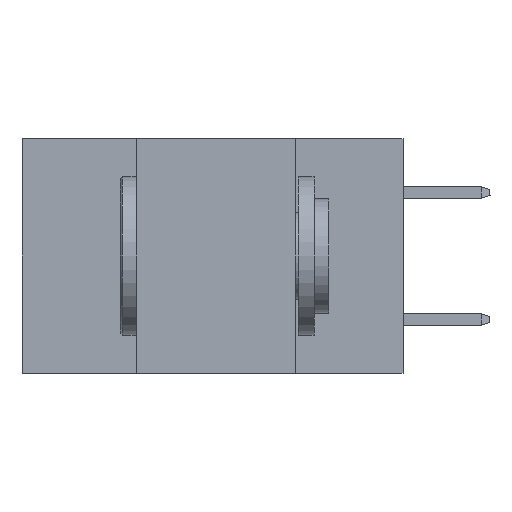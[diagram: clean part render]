
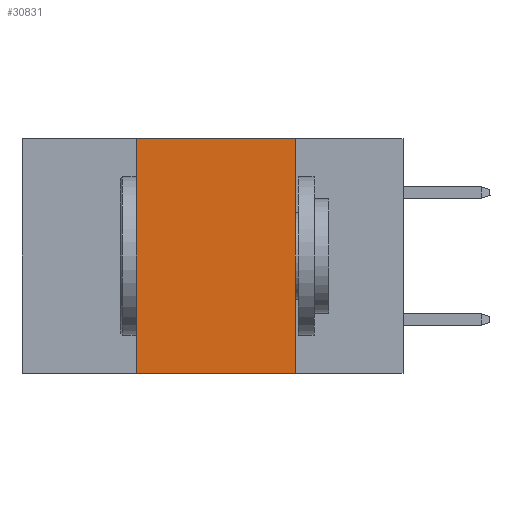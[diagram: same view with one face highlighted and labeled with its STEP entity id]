
A CAD part, left-side view. The second image highlights one B-rep face of the part: STEP entity #30831.
In plain terms, the highlighted planar face has unit normal (-1, 0, 0).
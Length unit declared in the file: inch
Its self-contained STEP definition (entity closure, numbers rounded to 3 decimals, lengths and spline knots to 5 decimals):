
#2144 = DIRECTION ( 'NONE',  ( 0., -1., 0. ) ) ;
#2482 = CARTESIAN_POINT ( 'NONE',  ( 0., 0.6, 0. ) ) ;
#2687 = DIRECTION ( 'NONE',  ( 1., 0., 0. ) ) ;
#2894 = PLANE ( 'NONE',  #32822 ) ;
#4077 = VECTOR ( 'NONE', #2144, 39.37008 ) ;
#4418 = CARTESIAN_POINT ( 'NONE',  ( 0., 0.17, -0.37 ) ) ;
#5688 = DIRECTION ( 'NONE',  ( 0., 0., 1. ) ) ;
#5837 = VECTOR ( 'NONE', #7224, 39.37008 ) ;
#6856 = EDGE_CURVE ( 'NONE', #21962, #34733, #12440, .T. ) ;
#7224 = DIRECTION ( 'NONE',  ( 0., 0., -1. ) ) ;
#7876 = CARTESIAN_POINT ( 'NONE',  ( 0., 0.6, -0.37 ) ) ;
#8128 = EDGE_CURVE ( 'NONE', #21962, #21107, #26295, .T. ) ;
#8427 = FACE_OUTER_BOUND ( 'NONE', #31121, .T. ) ;
#9967 = CARTESIAN_POINT ( 'NONE',  ( 0., 0.17, 0. ) ) ;
#10916 = ORIENTED_EDGE ( 'NONE', *, *, #25768, .F. ) ;
#11993 = ORIENTED_EDGE ( 'NONE', *, *, #35863, .F. ) ;
#12440 = LINE ( 'NONE', #18396, #23446 ) ;
#13232 = CARTESIAN_POINT ( 'NONE',  ( 0., 0.42, -0.37 ) ) ;
#16250 = LINE ( 'NONE', #25644, #5837 ) ;
#18396 = CARTESIAN_POINT ( 'NONE',  ( 0., 0.42, 0. ) ) ;
#18605 = LINE ( 'NONE', #37562, #29808 ) ;
#21107 = VERTEX_POINT ( 'NONE', #4418 ) ;
#21135 = DIRECTION ( 'NONE',  ( 0., 0., -1. ) ) ;
#21881 = DIRECTION ( 'NONE',  ( 0., -1., 0. ) ) ;
#21962 = VERTEX_POINT ( 'NONE', #13232 ) ;
#22033 = VERTEX_POINT ( 'NONE', #9967 ) ;
#23446 = VECTOR ( 'NONE', #5688, 39.37008 ) ;
#25644 = CARTESIAN_POINT ( 'NONE',  ( 0., 0.17, 0. ) ) ;
#25768 = EDGE_CURVE ( 'NONE', #22033, #21107, #16250, .T. ) ;
#26295 = LINE ( 'NONE', #7876, #4077 ) ;
#28885 = ORIENTED_EDGE ( 'NONE', *, *, #8128, .T. ) ;
#29326 = CARTESIAN_POINT ( 'NONE',  ( 0., 0.42, 0. ) ) ;
#29808 = VECTOR ( 'NONE', #21881, 39.37008 ) ;
#30831 = ADVANCED_FACE ( 'NONE', ( #8427 ), #2894, .F. ) ;
#31121 = EDGE_LOOP ( 'NONE', ( #10916, #11993, #31201, #28885 ) ) ;
#31201 = ORIENTED_EDGE ( 'NONE', *, *, #6856, .F. ) ;
#32822 = AXIS2_PLACEMENT_3D ( 'NONE', #2482, #2687, #21135 ) ;
#34733 = VERTEX_POINT ( 'NONE', #29326 ) ;
#35863 = EDGE_CURVE ( 'NONE', #34733, #22033, #18605, .T. ) ;
#37562 = CARTESIAN_POINT ( 'NONE',  ( 0., 0.6, 0. ) ) ;
